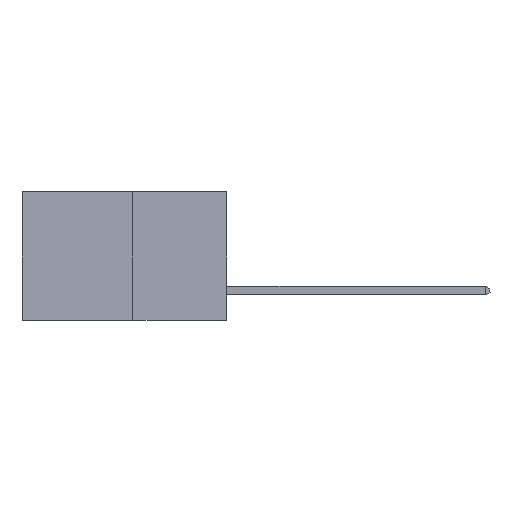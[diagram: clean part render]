
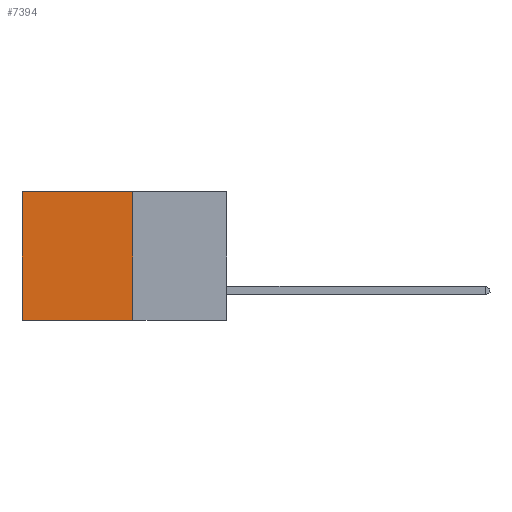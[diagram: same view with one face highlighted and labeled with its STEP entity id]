
A CAD part, left-side view. The second image highlights one B-rep face of the part: STEP entity #7394.
In plain terms, the highlighted planar face has unit normal (-1, 0, 0).
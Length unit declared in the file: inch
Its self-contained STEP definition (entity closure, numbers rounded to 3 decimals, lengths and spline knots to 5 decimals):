
#58 = LINE ( 'NONE', #10255, #10632 ) ;
#260 = DIRECTION ( 'NONE',  ( 0., 1., 0. ) ) ;
#724 = EDGE_CURVE ( 'NONE', #7278, #1844, #7651, .T. ) ;
#1026 = CARTESIAN_POINT ( 'NONE',  ( 0.277, 0.59, -0.37 ) ) ;
#1393 = EDGE_CURVE ( 'NONE', #1844, #1801, #9636, .T. ) ;
#1801 = VERTEX_POINT ( 'NONE', #1841 ) ;
#1841 = CARTESIAN_POINT ( 'NONE',  ( 0.277, 0.59, -0.37 ) ) ;
#1844 = VERTEX_POINT ( 'NONE', #5593 ) ;
#2589 = ORIENTED_EDGE ( 'NONE', *, *, #724, .T. ) ;
#2652 = CARTESIAN_POINT ( 'NONE',  ( 0.277, 0.27, -0.37 ) ) ;
#3084 = CARTESIAN_POINT ( 'NONE',  ( 0.277, 0.27, -0.37 ) ) ;
#3352 = VECTOR ( 'NONE', #4165, 39.37008 ) ;
#3666 = DIRECTION ( 'NONE',  ( 0., 1., 0. ) ) ;
#3669 = CARTESIAN_POINT ( 'NONE',  ( 0.277, 0.27, 0. ) ) ;
#4165 = DIRECTION ( 'NONE',  ( 0., 0., -1. ) ) ;
#4276 = CARTESIAN_POINT ( 'NONE',  ( 0.277, 0.27, -0.37 ) ) ;
#4308 = DIRECTION ( 'NONE',  ( 0., 0., -1. ) ) ;
#4337 = ORIENTED_EDGE ( 'NONE', *, *, #1393, .T. ) ;
#4340 = DIRECTION ( 'NONE',  ( 0., 0., -1. ) ) ;
#4394 = VECTOR ( 'NONE', #3666, 39.37008 ) ;
#5593 = CARTESIAN_POINT ( 'NONE',  ( 0.277, 0.59, 0. ) ) ;
#5881 = EDGE_LOOP ( 'NONE', ( #4337, #10767, #9028, #2589 ) ) ;
#6172 = VECTOR ( 'NONE', #4340, 39.37008 ) ;
#7278 = VERTEX_POINT ( 'NONE', #10410 ) ;
#7394 = ADVANCED_FACE ( 'NONE', ( #10408 ), #10505, .F. ) ;
#7651 = LINE ( 'NONE', #3669, #4394 ) ;
#7916 = EDGE_CURVE ( 'NONE', #8676, #1801, #58, .T. ) ;
#8676 = VERTEX_POINT ( 'NONE', #3084 ) ;
#8754 = AXIS2_PLACEMENT_3D ( 'NONE', #4276, #9033, #4308 ) ;
#9028 = ORIENTED_EDGE ( 'NONE', *, *, #10041, .F. ) ;
#9033 = DIRECTION ( 'NONE',  ( 1., 0., 0. ) ) ;
#9636 = LINE ( 'NONE', #1026, #3352 ) ;
#10000 = LINE ( 'NONE', #2652, #6172 ) ;
#10041 = EDGE_CURVE ( 'NONE', #7278, #8676, #10000, .T. ) ;
#10255 = CARTESIAN_POINT ( 'NONE',  ( 0.277, 0.27, -0.37 ) ) ;
#10408 = FACE_OUTER_BOUND ( 'NONE', #5881, .T. ) ;
#10410 = CARTESIAN_POINT ( 'NONE',  ( 0.277, 0.27, 0. ) ) ;
#10505 = PLANE ( 'NONE',  #8754 ) ;
#10632 = VECTOR ( 'NONE', #260, 39.37008 ) ;
#10767 = ORIENTED_EDGE ( 'NONE', *, *, #7916, .F. ) ;
